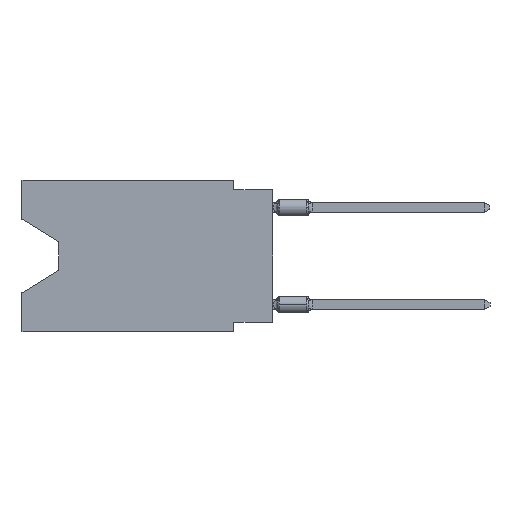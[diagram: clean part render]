
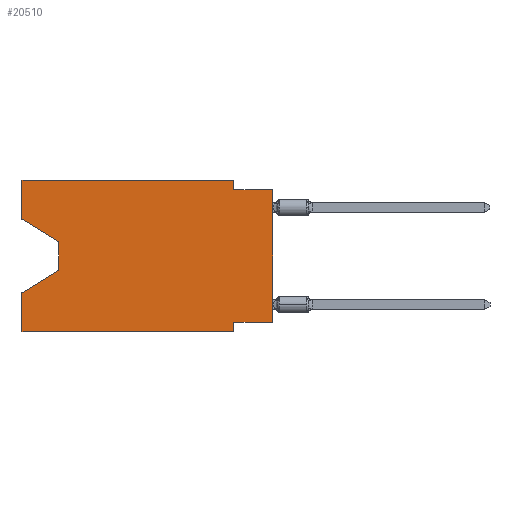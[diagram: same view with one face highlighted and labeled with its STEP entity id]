
A CAD part, left-side view. The second image highlights one B-rep face of the part: STEP entity #20510.
In plain terms, the highlighted planar face has unit normal (-1, 0, 0).
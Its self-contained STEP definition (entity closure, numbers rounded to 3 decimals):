
#48 = CARTESIAN_POINT ( 'NONE',  ( 0., 16.383, 0. ) ) ;
#221 = ORIENTED_EDGE ( 'NONE', *, *, #20262, .F. ) ;
#228 = CARTESIAN_POINT ( 'NONE',  ( 0., 2.54, 0. ) ) ;
#657 = VERTEX_POINT ( 'NONE', #30266 ) ;
#772 = AXIS2_PLACEMENT_3D ( 'NONE', #11853, #29040, #7721 ) ;
#1372 = VECTOR ( 'NONE', #19157, 1000. ) ;
#1733 = VECTOR ( 'NONE', #8910, 1000. ) ;
#1964 = CARTESIAN_POINT ( 'NONE',  ( 0., 13.97, -4.013 ) ) ;
#2041 = FACE_OUTER_BOUND ( 'NONE', #12105, .T. ) ;
#2096 = CARTESIAN_POINT ( 'NONE',  ( 0., 0., -0.635 ) ) ;
#2428 = VECTOR ( 'NONE', #25374, 1000. ) ;
#2472 = VERTEX_POINT ( 'NONE', #8159 ) ;
#2525 = EDGE_CURVE ( 'NONE', #2472, #12715, #29304, .T. ) ;
#3301 = VERTEX_POINT ( 'NONE', #28877 ) ;
#3620 = VERTEX_POINT ( 'NONE', #17989 ) ;
#4022 = VERTEX_POINT ( 'NONE', #26183 ) ;
#5523 = DIRECTION ( 'NONE',  ( 0., 0., -1. ) ) ;
#6113 = ORIENTED_EDGE ( 'NONE', *, *, #9273, .F. ) ;
#6462 = DIRECTION ( 'NONE',  ( 0., 1., 0. ) ) ;
#6959 = CARTESIAN_POINT ( 'NONE',  ( 0., 16.383, 0. ) ) ;
#6985 = CARTESIAN_POINT ( 'NONE',  ( 0., 0., -0.635 ) ) ;
#7200 = DIRECTION ( 'NONE',  ( 0., 0., 1. ) ) ;
#7532 = ORIENTED_EDGE ( 'NONE', *, *, #31705, .F. ) ;
#7595 = EDGE_CURVE ( 'NONE', #24784, #657, #24430, .T. ) ;
#7721 = DIRECTION ( 'NONE',  ( 0., 0., -1. ) ) ;
#7922 = ORIENTED_EDGE ( 'NONE', *, *, #24997, .F. ) ;
#7994 = VECTOR ( 'NONE', #30365, 1000. ) ;
#8159 = CARTESIAN_POINT ( 'NONE',  ( 0., 2.54, 0. ) ) ;
#8390 = ORIENTED_EDGE ( 'NONE', *, *, #2525, .F. ) ;
#8910 = DIRECTION ( 'NONE',  ( 0., 0., 1. ) ) ;
#9075 = LINE ( 'NONE', #11650, #1733 ) ;
#9273 = EDGE_CURVE ( 'NONE', #3620, #32783, #26040, .T. ) ;
#9558 = LINE ( 'NONE', #6985, #15133 ) ;
#9804 = VERTEX_POINT ( 'NONE', #23754 ) ;
#10179 = VECTOR ( 'NONE', #33090, 1000. ) ;
#10252 = DIRECTION ( 'NONE',  ( 0., -1., 0. ) ) ;
#10309 = VERTEX_POINT ( 'NONE', #28879 ) ;
#10759 = ORIENTED_EDGE ( 'NONE', *, *, #23859, .F. ) ;
#11650 = CARTESIAN_POINT ( 'NONE',  ( 0., 16.383, 0. ) ) ;
#11853 = CARTESIAN_POINT ( 'NONE',  ( 0., 16.383, 0. ) ) ;
#12073 = EDGE_CURVE ( 'NONE', #4022, #10309, #16437, .T. ) ;
#12105 = EDGE_LOOP ( 'NONE', ( #15217, #25660, #22710, #7532, #19991, #221, #30982, #23904, #10759, #8390, #7922, #6113 ) ) ;
#12355 = PLANE ( 'NONE',  #772 ) ;
#12715 = VERTEX_POINT ( 'NONE', #25494 ) ;
#12878 = VECTOR ( 'NONE', #23748, 1000. ) ;
#13249 = CARTESIAN_POINT ( 'NONE',  ( 0., 2.54, -9.906 ) ) ;
#13434 = CARTESIAN_POINT ( 'NONE',  ( 0., 16.383, -2.546 ) ) ;
#13529 = VECTOR ( 'NONE', #21041, 1000. ) ;
#14608 = CARTESIAN_POINT ( 'NONE',  ( 0., 0., 0. ) ) ;
#14927 = VERTEX_POINT ( 'NONE', #21416 ) ;
#15039 = LINE ( 'NONE', #25528, #10179 ) ;
#15066 = DIRECTION ( 'NONE',  ( 0., -0.855, -0.519 ) ) ;
#15133 = VECTOR ( 'NONE', #10252, 1000. ) ;
#15217 = ORIENTED_EDGE ( 'NONE', *, *, #32250, .T. ) ;
#15457 = VECTOR ( 'NONE', #7200, 1000. ) ;
#15497 = VECTOR ( 'NONE', #15066, 1000. ) ;
#15508 = LINE ( 'NONE', #13249, #12878 ) ;
#15980 = VECTOR ( 'NONE', #5523, 1000. ) ;
#16437 = LINE ( 'NONE', #26932, #16668 ) ;
#16668 = VECTOR ( 'NONE', #6462, 1000. ) ;
#17816 = LINE ( 'NONE', #13434, #15497 ) ;
#17989 = CARTESIAN_POINT ( 'NONE',  ( 0., 16.383, -2.546 ) ) ;
#19157 = DIRECTION ( 'NONE',  ( 0., 0., -1. ) ) ;
#19219 = EDGE_CURVE ( 'NONE', #4022, #30954, #30267, .T. ) ;
#19991 = ORIENTED_EDGE ( 'NONE', *, *, #25951, .T. ) ;
#20262 = EDGE_CURVE ( 'NONE', #10309, #14927, #15508, .T. ) ;
#20510 = ADVANCED_FACE ( 'NONE', ( #2041 ), #12355, .F. ) ;
#21041 = DIRECTION ( 'NONE',  ( 0., -1., 0. ) ) ;
#21416 = CARTESIAN_POINT ( 'NONE',  ( 0., 2.54, -9.906 ) ) ;
#22273 = LINE ( 'NONE', #33104, #7994 ) ;
#22710 = ORIENTED_EDGE ( 'NONE', *, *, #23077, .T. ) ;
#23077 = EDGE_CURVE ( 'NONE', #657, #9804, #15039, .T. ) ;
#23748 = DIRECTION ( 'NONE',  ( 0., 0., -1. ) ) ;
#23754 = CARTESIAN_POINT ( 'NONE',  ( 0., 16.383, -7.36 ) ) ;
#23859 = EDGE_CURVE ( 'NONE', #12715, #30954, #9558, .T. ) ;
#23904 = ORIENTED_EDGE ( 'NONE', *, *, #19219, .T. ) ;
#24098 = CARTESIAN_POINT ( 'NONE',  ( 0., 13.97, -4.013 ) ) ;
#24430 = LINE ( 'NONE', #24098, #15980 ) ;
#24784 = VERTEX_POINT ( 'NONE', #1964 ) ;
#24997 = EDGE_CURVE ( 'NONE', #32783, #2472, #32034, .T. ) ;
#25374 = DIRECTION ( 'NONE',  ( 0., 0., 1. ) ) ;
#25494 = CARTESIAN_POINT ( 'NONE',  ( 0., 2.54, -0.635 ) ) ;
#25528 = CARTESIAN_POINT ( 'NONE',  ( 0., 13.97, -5.893 ) ) ;
#25660 = ORIENTED_EDGE ( 'NONE', *, *, #7595, .T. ) ;
#25951 = EDGE_CURVE ( 'NONE', #3301, #14927, #22273, .T. ) ;
#26040 = LINE ( 'NONE', #6959, #2428 ) ;
#26183 = CARTESIAN_POINT ( 'NONE',  ( 0., 0., -9.271 ) ) ;
#26932 = CARTESIAN_POINT ( 'NONE',  ( 0., 0., -9.271 ) ) ;
#28636 = CARTESIAN_POINT ( 'NONE',  ( 0., 16.383, 0. ) ) ;
#28877 = CARTESIAN_POINT ( 'NONE',  ( 0., 16.383, -9.906 ) ) ;
#28879 = CARTESIAN_POINT ( 'NONE',  ( 0., 2.54, -9.271 ) ) ;
#29040 = DIRECTION ( 'NONE',  ( 1., 0., 0. ) ) ;
#29304 = LINE ( 'NONE', #228, #1372 ) ;
#30266 = CARTESIAN_POINT ( 'NONE',  ( 0., 13.97, -5.893 ) ) ;
#30267 = LINE ( 'NONE', #14608, #15457 ) ;
#30365 = DIRECTION ( 'NONE',  ( 0., -1., 0. ) ) ;
#30954 = VERTEX_POINT ( 'NONE', #2096 ) ;
#30982 = ORIENTED_EDGE ( 'NONE', *, *, #12073, .F. ) ;
#31705 = EDGE_CURVE ( 'NONE', #3301, #9804, #9075, .T. ) ;
#32034 = LINE ( 'NONE', #48, #13529 ) ;
#32250 = EDGE_CURVE ( 'NONE', #3620, #24784, #17816, .T. ) ;
#32783 = VERTEX_POINT ( 'NONE', #28636 ) ;
#33090 = DIRECTION ( 'NONE',  ( 0., 0.855, -0.519 ) ) ;
#33104 = CARTESIAN_POINT ( 'NONE',  ( 0., 16.383, -9.906 ) ) ;
